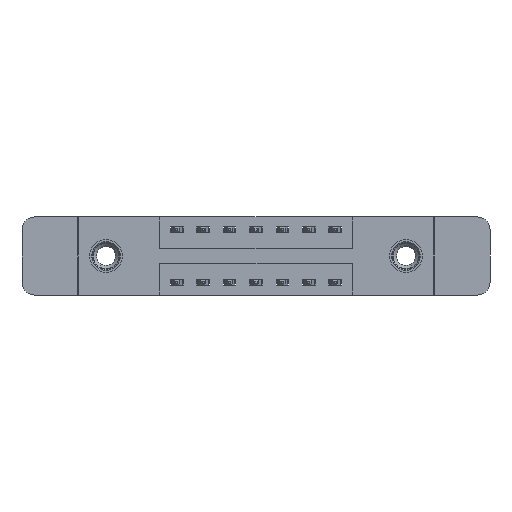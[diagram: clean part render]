
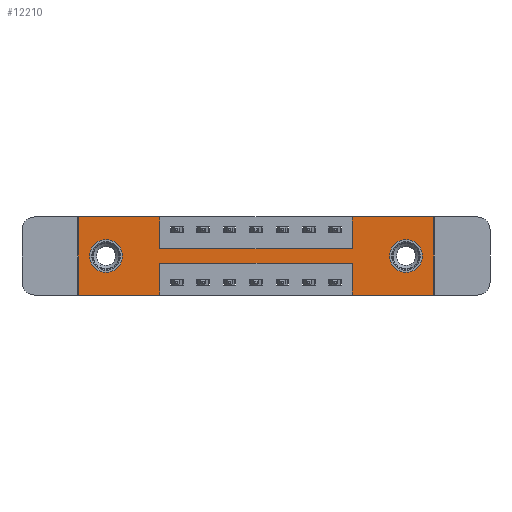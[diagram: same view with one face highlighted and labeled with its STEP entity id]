
A CAD part, front view. The second image highlights one B-rep face of the part: STEP entity #12210.
In plain terms, the highlighted planar face has unit normal (0, -1, 0).
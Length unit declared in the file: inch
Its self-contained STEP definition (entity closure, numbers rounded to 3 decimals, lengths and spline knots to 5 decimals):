
#344 = VECTOR ( 'NONE', #7832, 39.37008 ) ;
#521 = ORIENTED_EDGE ( 'NONE', *, *, #11386, .F. ) ;
#561 = EDGE_CURVE ( 'NONE', #2636, #2738, #4760, .T. ) ;
#817 = EDGE_CURVE ( 'NONE', #10647, #2636, #5793, .T. ) ;
#834 = VECTOR ( 'NONE', #2042, 39.37008 ) ;
#983 = EDGE_CURVE ( 'NONE', #7680, #9721, #7368, .T. ) ;
#1026 = LINE ( 'NONE', #11020, #834 ) ;
#1180 = EDGE_CURVE ( 'NONE', #2738, #10677, #5777, .T. ) ;
#1197 = FACE_BOUND ( 'NONE', #3220, .T. ) ;
#1316 = AXIS2_PLACEMENT_3D ( 'NONE', #7193, #12739, #10428 ) ;
#1469 = ORIENTED_EDGE ( 'NONE', *, *, #4240, .T. ) ;
#1523 = EDGE_LOOP ( 'NONE', ( #5137, #1600 ) ) ;
#1600 = ORIENTED_EDGE ( 'NONE', *, *, #8667, .T. ) ;
#1717 = VERTEX_POINT ( 'NONE', #10869 ) ;
#1722 = CARTESIAN_POINT ( 'NONE',  ( 0., 0., 0. ) ) ;
#1735 = CARTESIAN_POINT ( 'NONE',  ( 0., 0., 0. ) ) ;
#1828 = DIRECTION ( 'NONE',  ( 0., 0., -1. ) ) ;
#1987 = VERTEX_POINT ( 'NONE', #4044 ) ;
#2042 = DIRECTION ( 'NONE',  ( -1., 0., 0. ) ) ;
#2350 = LINE ( 'NONE', #1722, #9715 ) ;
#2429 = ORIENTED_EDGE ( 'NONE', *, *, #4854, .F. ) ;
#2536 = DIRECTION ( 'NONE',  ( 0., 0., -1. ) ) ;
#2636 = VERTEX_POINT ( 'NONE', #13415 ) ;
#2738 = VERTEX_POINT ( 'NONE', #11394 ) ;
#2763 = CARTESIAN_POINT ( 'NONE',  ( 0.1325, 0., -0.185 ) ) ;
#2795 = CARTESIAN_POINT ( 'NONE',  ( 0., 0., 0. ) ) ;
#2949 = FACE_BOUND ( 'NONE', #1523, .T. ) ;
#3220 = EDGE_LOOP ( 'NONE', ( #7091, #1469 ) ) ;
#3253 = EDGE_CURVE ( 'NONE', #10677, #5749, #5197, .T. ) ;
#3610 = CARTESIAN_POINT ( 'NONE',  ( 0.3875, 0., -0.22 ) ) ;
#3731 = EDGE_CURVE ( 'NONE', #5749, #11164, #10789, .T. ) ;
#3732 = CARTESIAN_POINT ( 'NONE',  ( 0., 0., -0.37 ) ) ;
#3761 = CARTESIAN_POINT ( 'NONE',  ( 0.3875, 0., 0. ) ) ;
#3969 = LINE ( 'NONE', #12702, #12548 ) ;
#4044 = CARTESIAN_POINT ( 'NONE',  ( 0., 0., -0.37 ) ) ;
#4240 = EDGE_CURVE ( 'NONE', #8388, #6624, #8498, .T. ) ;
#4371 = VECTOR ( 'NONE', #8804, 39.37008 ) ;
#4526 = EDGE_CURVE ( 'NONE', #6624, #8388, #9554, .T. ) ;
#4550 = EDGE_CURVE ( 'NONE', #1987, #5976, #2350, .T. ) ;
#4695 = PLANE ( 'NONE',  #1316 ) ;
#4760 = LINE ( 'NONE', #6958, #6327 ) ;
#4854 = EDGE_CURVE ( 'NONE', #9721, #1717, #10197, .T. ) ;
#4959 = CARTESIAN_POINT ( 'NONE',  ( 1.5525, 0., -0.185 ) ) ;
#5137 = ORIENTED_EDGE ( 'NONE', *, *, #8774, .T. ) ;
#5161 = DIRECTION ( 'NONE',  ( 1., 0., 0. ) ) ;
#5197 = LINE ( 'NONE', #7445, #7834 ) ;
#5299 = DIRECTION ( 'NONE',  ( 0., 0., -1. ) ) ;
#5400 = CARTESIAN_POINT ( 'NONE',  ( 0., 0., 0. ) ) ;
#5599 = CARTESIAN_POINT ( 'NONE',  ( 0.1325, 0., -0.107 ) ) ;
#5749 = VERTEX_POINT ( 'NONE', #12115 ) ;
#5777 = LINE ( 'NONE', #3732, #13991 ) ;
#5793 = LINE ( 'NONE', #1735, #11047 ) ;
#5825 = CIRCLE ( 'NONE', #8500, 0.078 ) ;
#5888 = ORIENTED_EDGE ( 'NONE', *, *, #13080, .F. ) ;
#5974 = ORIENTED_EDGE ( 'NONE', *, *, #3253, .F. ) ;
#5976 = VERTEX_POINT ( 'NONE', #2795 ) ;
#6128 = DIRECTION ( 'NONE',  ( 0., 1., 0. ) ) ;
#6174 = DIRECTION ( 'NONE',  ( 0., 0., -1. ) ) ;
#6220 = DIRECTION ( 'NONE',  ( 0., 1., 0. ) ) ;
#6224 = VECTOR ( 'NONE', #13623, 39.37008 ) ;
#6327 = VECTOR ( 'NONE', #13736, 39.37008 ) ;
#6624 = VERTEX_POINT ( 'NONE', #5599 ) ;
#6843 = VERTEX_POINT ( 'NONE', #11259 ) ;
#6958 = CARTESIAN_POINT ( 'NONE',  ( 1.685, 0., 0. ) ) ;
#7091 = ORIENTED_EDGE ( 'NONE', *, *, #4526, .T. ) ;
#7193 = CARTESIAN_POINT ( 'NONE',  ( 0., 0., -0.37 ) ) ;
#7270 = VECTOR ( 'NONE', #11545, 39.37008 ) ;
#7353 = LINE ( 'NONE', #12221, #4371 ) ;
#7368 = LINE ( 'NONE', #3761, #9290 ) ;
#7384 = CARTESIAN_POINT ( 'NONE',  ( 0.3875, 0., 0. ) ) ;
#7445 = CARTESIAN_POINT ( 'NONE',  ( 1.2975, 0., -0.37 ) ) ;
#7680 = VERTEX_POINT ( 'NONE', #7384 ) ;
#7832 = DIRECTION ( 'NONE',  ( 1., 0., 0. ) ) ;
#7834 = VECTOR ( 'NONE', #14087, 39.37008 ) ;
#7943 = CARTESIAN_POINT ( 'NONE',  ( 0.1325, 0., -0.263 ) ) ;
#8388 = VERTEX_POINT ( 'NONE', #7943 ) ;
#8438 = CARTESIAN_POINT ( 'NONE',  ( 0.1325, 0., -0.185 ) ) ;
#8498 = CIRCLE ( 'NONE', #13957, 0.078 ) ;
#8500 = AXIS2_PLACEMENT_3D ( 'NONE', #4959, #6220, #6174 ) ;
#8667 = EDGE_CURVE ( 'NONE', #11815, #6843, #5825, .T. ) ;
#8731 = ORIENTED_EDGE ( 'NONE', *, *, #11567, .F. ) ;
#8774 = EDGE_CURVE ( 'NONE', #6843, #11815, #10015, .T. ) ;
#8804 = DIRECTION ( 'NONE',  ( 0., 0., 1. ) ) ;
#9084 = CARTESIAN_POINT ( 'NONE',  ( 1.5525, 0., -0.263 ) ) ;
#9290 = VECTOR ( 'NONE', #1828, 39.37008 ) ;
#9537 = DIRECTION ( 'NONE',  ( 0., 0., 1. ) ) ;
#9554 = CIRCLE ( 'NONE', #10038, 0.078 ) ;
#9715 = VECTOR ( 'NONE', #13993, 39.37008 ) ;
#9721 = VERTEX_POINT ( 'NONE', #13930 ) ;
#9778 = DIRECTION ( 'NONE',  ( 0., 1., 0. ) ) ;
#9937 = ORIENTED_EDGE ( 'NONE', *, *, #12572, .F. ) ;
#9947 = VERTEX_POINT ( 'NONE', #14489 ) ;
#9965 = LINE ( 'NONE', #5400, #344 ) ;
#10015 = CIRCLE ( 'NONE', #12693, 0.078 ) ;
#10038 = AXIS2_PLACEMENT_3D ( 'NONE', #8438, #6128, #13941 ) ;
#10197 = LINE ( 'NONE', #13575, #7270 ) ;
#10224 = CARTESIAN_POINT ( 'NONE',  ( 0.3875, 0., -0.22 ) ) ;
#10290 = CARTESIAN_POINT ( 'NONE',  ( 1.2975, 0., 0. ) ) ;
#10428 = DIRECTION ( 'NONE',  ( 0., 0., -1. ) ) ;
#10486 = DIRECTION ( 'NONE',  ( 0., 1., 0. ) ) ;
#10647 = VERTEX_POINT ( 'NONE', #10290 ) ;
#10677 = VERTEX_POINT ( 'NONE', #12422 ) ;
#10789 = LINE ( 'NONE', #10224, #6224 ) ;
#10869 = CARTESIAN_POINT ( 'NONE',  ( 1.2975, 0., -0.15 ) ) ;
#11020 = CARTESIAN_POINT ( 'NONE',  ( 0., 0., -0.37 ) ) ;
#11047 = VECTOR ( 'NONE', #5161, 39.37008 ) ;
#11164 = VERTEX_POINT ( 'NONE', #3610 ) ;
#11259 = CARTESIAN_POINT ( 'NONE',  ( 1.5525, 0., -0.107 ) ) ;
#11313 = EDGE_LOOP ( 'NONE', ( #5888, #13725, #5974, #13812, #13647, #12998, #8731, #2429, #12918, #521, #13480, #9937 ) ) ;
#11386 = EDGE_CURVE ( 'NONE', #5976, #7680, #9965, .T. ) ;
#11394 = CARTESIAN_POINT ( 'NONE',  ( 1.685, 0., -0.37 ) ) ;
#11506 = FACE_OUTER_BOUND ( 'NONE', #11313, .T. ) ;
#11545 = DIRECTION ( 'NONE',  ( 1., 0., 0. ) ) ;
#11567 = EDGE_CURVE ( 'NONE', #1717, #10647, #7353, .T. ) ;
#11617 = DIRECTION ( 'NONE',  ( -1., 0., 0. ) ) ;
#11815 = VERTEX_POINT ( 'NONE', #9084 ) ;
#12115 = CARTESIAN_POINT ( 'NONE',  ( 1.2975, 0., -0.22 ) ) ;
#12210 = ADVANCED_FACE ( 'NONE', ( #2949, #1197, #11506 ), #4695, .T. ) ;
#12221 = CARTESIAN_POINT ( 'NONE',  ( 1.2975, 0., 0. ) ) ;
#12422 = CARTESIAN_POINT ( 'NONE',  ( 1.2975, 0., -0.37 ) ) ;
#12548 = VECTOR ( 'NONE', #2536, 39.37008 ) ;
#12572 = EDGE_CURVE ( 'NONE', #9947, #1987, #1026, .T. ) ;
#12693 = AXIS2_PLACEMENT_3D ( 'NONE', #14131, #9778, #5299 ) ;
#12702 = CARTESIAN_POINT ( 'NONE',  ( 0.3875, 0., -0.37 ) ) ;
#12739 = DIRECTION ( 'NONE',  ( 0., -1., 0. ) ) ;
#12918 = ORIENTED_EDGE ( 'NONE', *, *, #983, .F. ) ;
#12998 = ORIENTED_EDGE ( 'NONE', *, *, #817, .F. ) ;
#13080 = EDGE_CURVE ( 'NONE', #11164, #9947, #3969, .T. ) ;
#13415 = CARTESIAN_POINT ( 'NONE',  ( 1.685, 0., 0. ) ) ;
#13480 = ORIENTED_EDGE ( 'NONE', *, *, #4550, .F. ) ;
#13575 = CARTESIAN_POINT ( 'NONE',  ( 0.3875, 0., -0.15 ) ) ;
#13623 = DIRECTION ( 'NONE',  ( -1., 0., 0. ) ) ;
#13647 = ORIENTED_EDGE ( 'NONE', *, *, #561, .F. ) ;
#13725 = ORIENTED_EDGE ( 'NONE', *, *, #3731, .F. ) ;
#13736 = DIRECTION ( 'NONE',  ( 0., 0., -1. ) ) ;
#13812 = ORIENTED_EDGE ( 'NONE', *, *, #1180, .F. ) ;
#13930 = CARTESIAN_POINT ( 'NONE',  ( 0.3875, 0., -0.15 ) ) ;
#13941 = DIRECTION ( 'NONE',  ( 0., 0., 1. ) ) ;
#13957 = AXIS2_PLACEMENT_3D ( 'NONE', #2763, #10486, #9537 ) ;
#13991 = VECTOR ( 'NONE', #11617, 39.37008 ) ;
#13993 = DIRECTION ( 'NONE',  ( 0., 0., 1. ) ) ;
#14087 = DIRECTION ( 'NONE',  ( 0., 0., 1. ) ) ;
#14131 = CARTESIAN_POINT ( 'NONE',  ( 1.5525, 0., -0.185 ) ) ;
#14489 = CARTESIAN_POINT ( 'NONE',  ( 0.3875, 0., -0.37 ) ) ;
